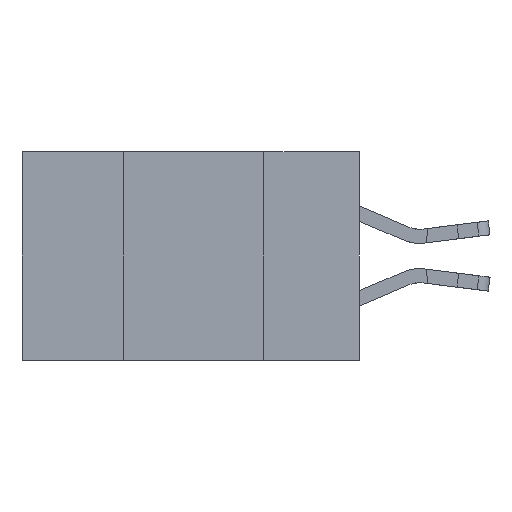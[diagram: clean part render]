
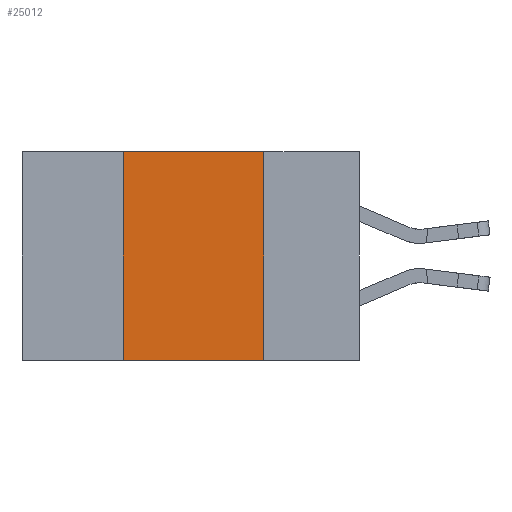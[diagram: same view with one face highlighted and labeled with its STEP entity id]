
A CAD part, left-side view. The second image highlights one B-rep face of the part: STEP entity #25012.
In plain terms, the highlighted planar face has unit normal (-1, 0, 0).
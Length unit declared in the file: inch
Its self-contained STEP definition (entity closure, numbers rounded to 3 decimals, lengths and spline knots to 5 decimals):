
#995 = VERTEX_POINT ( 'NONE', #9101 ) ;
#2009 = CARTESIAN_POINT ( 'NONE',  ( 0., 0.17, -0.37 ) ) ;
#2654 = CARTESIAN_POINT ( 'NONE',  ( 0., 0.17, 0. ) ) ;
#3185 = ORIENTED_EDGE ( 'NONE', *, *, #22752, .T. ) ;
#3943 = CARTESIAN_POINT ( 'NONE',  ( 0., 0.6, -0.37 ) ) ;
#3992 = DIRECTION ( 'NONE',  ( 0., 0., -1. ) ) ;
#4138 = AXIS2_PLACEMENT_3D ( 'NONE', #17231, #17405, #9339 ) ;
#4286 = ORIENTED_EDGE ( 'NONE', *, *, #10142, .F. ) ;
#4698 = LINE ( 'NONE', #5076, #8811 ) ;
#5076 = CARTESIAN_POINT ( 'NONE',  ( 0., 0.6, 0. ) ) ;
#5336 = DIRECTION ( 'NONE',  ( 0., -1., 0. ) ) ;
#5692 = CARTESIAN_POINT ( 'NONE',  ( 0., 0.42, -0.37 ) ) ;
#6238 = EDGE_LOOP ( 'NONE', ( #4286, #16155, #9170, #3185 ) ) ;
#8738 = VECTOR ( 'NONE', #3992, 39.37008 ) ;
#8811 = VECTOR ( 'NONE', #5336, 39.37008 ) ;
#8837 = EDGE_CURVE ( 'NONE', #995, #23437, #4698, .T. ) ;
#8936 = VERTEX_POINT ( 'NONE', #5692 ) ;
#9101 = CARTESIAN_POINT ( 'NONE',  ( 0., 0.42, 0. ) ) ;
#9170 = ORIENTED_EDGE ( 'NONE', *, *, #23731, .F. ) ;
#9339 = DIRECTION ( 'NONE',  ( 0., 0., -1. ) ) ;
#10142 = EDGE_CURVE ( 'NONE', #23437, #17546, #21745, .T. ) ;
#13315 = CARTESIAN_POINT ( 'NONE',  ( 0., 0.42, 0. ) ) ;
#13373 = VECTOR ( 'NONE', #23511, 39.37008 ) ;
#15366 = PLANE ( 'NONE',  #4138 ) ;
#16155 = ORIENTED_EDGE ( 'NONE', *, *, #8837, .F. ) ;
#16768 = FACE_OUTER_BOUND ( 'NONE', #6238, .T. ) ;
#17070 = LINE ( 'NONE', #3943, #22515 ) ;
#17231 = CARTESIAN_POINT ( 'NONE',  ( 0., 0.6, 0. ) ) ;
#17405 = DIRECTION ( 'NONE',  ( 1., 0., 0. ) ) ;
#17546 = VERTEX_POINT ( 'NONE', #2009 ) ;
#18134 = DIRECTION ( 'NONE',  ( 0., -1., 0. ) ) ;
#20142 = CARTESIAN_POINT ( 'NONE',  ( 0., 0.17, 0. ) ) ;
#20988 = LINE ( 'NONE', #13315, #13373 ) ;
#21745 = LINE ( 'NONE', #20142, #8738 ) ;
#22515 = VECTOR ( 'NONE', #18134, 39.37008 ) ;
#22752 = EDGE_CURVE ( 'NONE', #8936, #17546, #17070, .T. ) ;
#23437 = VERTEX_POINT ( 'NONE', #2654 ) ;
#23511 = DIRECTION ( 'NONE',  ( 0., 0., 1. ) ) ;
#23731 = EDGE_CURVE ( 'NONE', #8936, #995, #20988, .T. ) ;
#25012 = ADVANCED_FACE ( 'NONE', ( #16768 ), #15366, .F. ) ;
